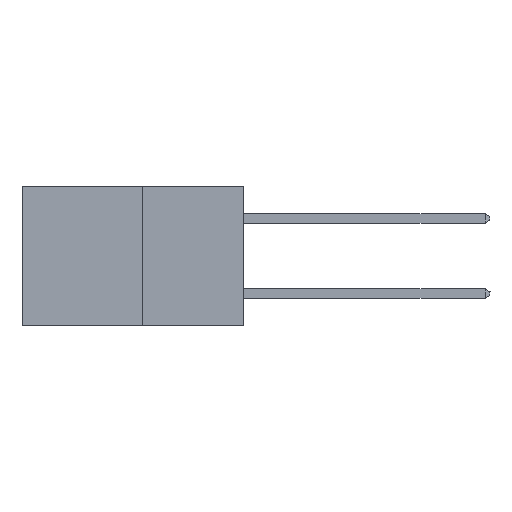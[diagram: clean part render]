
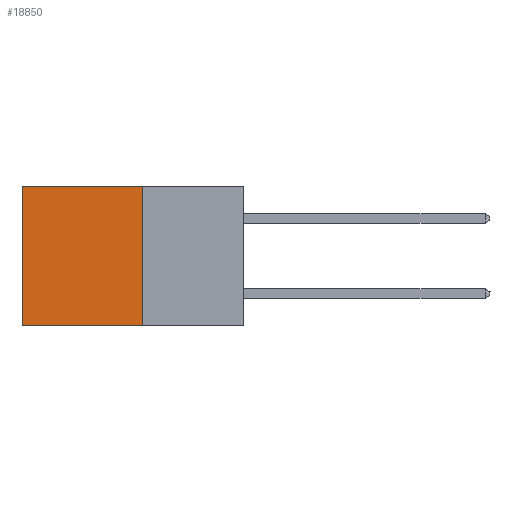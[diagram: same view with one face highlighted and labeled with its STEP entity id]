
A CAD part, left-side view. The second image highlights one B-rep face of the part: STEP entity #18850.
In plain terms, the highlighted planar face has unit normal (-1, 0, 0).
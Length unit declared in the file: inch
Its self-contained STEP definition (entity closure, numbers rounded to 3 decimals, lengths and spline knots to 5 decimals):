
#329 = DIRECTION ( 'NONE',  ( 0., 0., -1. ) ) ;
#1846 = VECTOR ( 'NONE', #25689, 39.37008 ) ;
#1966 = DIRECTION ( 'NONE',  ( 0., 0., -1. ) ) ;
#3192 = VECTOR ( 'NONE', #329, 39.37008 ) ;
#5753 = CARTESIAN_POINT ( 'NONE',  ( 0.277, 0.59, -0.37 ) ) ;
#7191 = CARTESIAN_POINT ( 'NONE',  ( 0.277, 0.59, -0.37 ) ) ;
#7273 = DIRECTION ( 'NONE',  ( 0., 1., 0. ) ) ;
#8861 = VERTEX_POINT ( 'NONE', #14113 ) ;
#8898 = CARTESIAN_POINT ( 'NONE',  ( 0.277, 0.27, -0.37 ) ) ;
#10145 = LINE ( 'NONE', #31477, #3192 ) ;
#10545 = ORIENTED_EDGE ( 'NONE', *, *, #33666, .T. ) ;
#10803 = CARTESIAN_POINT ( 'NONE',  ( 0.277, 0.27, -0.37 ) ) ;
#12264 = VECTOR ( 'NONE', #7273, 39.37008 ) ;
#13205 = VERTEX_POINT ( 'NONE', #5753 ) ;
#14113 = CARTESIAN_POINT ( 'NONE',  ( 0.277, 0.27, 0. ) ) ;
#15450 = ORIENTED_EDGE ( 'NONE', *, *, #17950, .T. ) ;
#16042 = DIRECTION ( 'NONE',  ( 0., 0., -1. ) ) ;
#16493 = ORIENTED_EDGE ( 'NONE', *, *, #18625, .F. ) ;
#17346 = LINE ( 'NONE', #23172, #1846 ) ;
#17950 = EDGE_CURVE ( 'NONE', #25701, #13205, #33072, .T. ) ;
#18625 = EDGE_CURVE ( 'NONE', #32663, #13205, #32271, .T. ) ;
#18793 = FACE_OUTER_BOUND ( 'NONE', #29490, .T. ) ;
#18850 = ADVANCED_FACE ( 'NONE', ( #18793 ), #26497, .F. ) ;
#21289 = AXIS2_PLACEMENT_3D ( 'NONE', #10803, #31697, #16042 ) ;
#23172 = CARTESIAN_POINT ( 'NONE',  ( 0.277, 0.27, 0. ) ) ;
#25386 = VECTOR ( 'NONE', #1966, 39.37008 ) ;
#25590 = CARTESIAN_POINT ( 'NONE',  ( 0.277, 0.27, -0.37 ) ) ;
#25689 = DIRECTION ( 'NONE',  ( 0., 1., 0. ) ) ;
#25701 = VERTEX_POINT ( 'NONE', #30810 ) ;
#26497 = PLANE ( 'NONE',  #21289 ) ;
#29490 = EDGE_LOOP ( 'NONE', ( #15450, #16493, #30953, #10545 ) ) ;
#30810 = CARTESIAN_POINT ( 'NONE',  ( 0.277, 0.59, 0. ) ) ;
#30953 = ORIENTED_EDGE ( 'NONE', *, *, #31008, .F. ) ;
#31008 = EDGE_CURVE ( 'NONE', #8861, #32663, #10145, .T. ) ;
#31477 = CARTESIAN_POINT ( 'NONE',  ( 0.277, 0.27, -0.37 ) ) ;
#31697 = DIRECTION ( 'NONE',  ( 1., 0., 0. ) ) ;
#32271 = LINE ( 'NONE', #25590, #12264 ) ;
#32663 = VERTEX_POINT ( 'NONE', #8898 ) ;
#33072 = LINE ( 'NONE', #7191, #25386 ) ;
#33666 = EDGE_CURVE ( 'NONE', #8861, #25701, #17346, .T. ) ;
